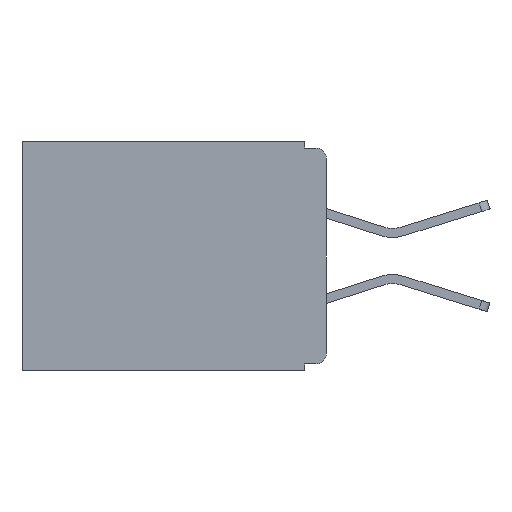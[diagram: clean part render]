
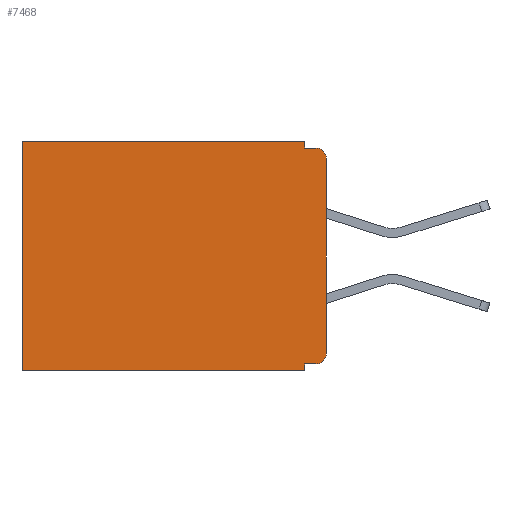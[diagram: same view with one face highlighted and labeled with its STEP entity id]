
A CAD part, left-side view. The second image highlights one B-rep face of the part: STEP entity #7468.
In plain terms, the highlighted planar face has unit normal (-1, 0, 0).
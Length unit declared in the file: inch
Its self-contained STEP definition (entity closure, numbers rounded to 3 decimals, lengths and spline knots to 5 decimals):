
#40 = CARTESIAN_POINT ( 'NONE',  ( 0.3, 0., -0.33 ) ) ;
#110 = CARTESIAN_POINT ( 'NONE',  ( 0.3, 0., -0.33 ) ) ;
#550 = VERTEX_POINT ( 'NONE', #2138 ) ;
#823 = ORIENTED_EDGE ( 'NONE', *, *, #13228, .T. ) ;
#982 = AXIS2_PLACEMENT_3D ( 'NONE', #19298, #19705, #19097 ) ;
#1581 = ORIENTED_EDGE ( 'NONE', *, *, #14726, .F. ) ;
#1845 = CARTESIAN_POINT ( 'NONE',  ( 0.3, 0., -0.32 ) ) ;
#2033 = AXIS2_PLACEMENT_3D ( 'NONE', #8565, #28020, #26029 ) ;
#2046 = DIRECTION ( 'NONE',  ( 0., 0., -1. ) ) ;
#2138 = CARTESIAN_POINT ( 'NONE',  ( 0.3, 0., -0.025 ) ) ;
#2230 = CARTESIAN_POINT ( 'NONE',  ( 0.3, 0.031, 0. ) ) ;
#2409 = EDGE_CURVE ( 'NONE', #550, #13899, #5448, .T. ) ;
#3191 = EDGE_CURVE ( 'NONE', #550, #28279, #14592, .T. ) ;
#3737 = EDGE_CURVE ( 'NONE', #4046, #18161, #4598, .T. ) ;
#4046 = VERTEX_POINT ( 'NONE', #23439 ) ;
#4598 = LINE ( 'NONE', #6097, #22523 ) ;
#5448 = LINE ( 'NONE', #110, #29412 ) ;
#5674 = CARTESIAN_POINT ( 'NONE',  ( 0.3, 0., -0.01 ) ) ;
#5685 = ORIENTED_EDGE ( 'NONE', *, *, #8941, .F. ) ;
#6097 = CARTESIAN_POINT ( 'NONE',  ( 0.3, 0.437, -0.33 ) ) ;
#6102 = ORIENTED_EDGE ( 'NONE', *, *, #2409, .F. ) ;
#6124 = DIRECTION ( 'NONE',  ( 0., 0., -1. ) ) ;
#6241 = EDGE_CURVE ( 'NONE', #25258, #23703, #10054, .T. ) ;
#6731 = ORIENTED_EDGE ( 'NONE', *, *, #9348, .F. ) ;
#7194 = CARTESIAN_POINT ( 'NONE',  ( 0.3, 0.015, -0.305 ) ) ;
#7468 = ADVANCED_FACE ( 'NONE', ( #25947 ), #19167, .F. ) ;
#7916 = CARTESIAN_POINT ( 'NONE',  ( 0.3, 0.031, -0.01 ) ) ;
#8565 = CARTESIAN_POINT ( 'NONE',  ( 0.3, 0.015, -0.025 ) ) ;
#8941 = EDGE_CURVE ( 'NONE', #23141, #21134, #21333, .T. ) ;
#9329 = CARTESIAN_POINT ( 'NONE',  ( 0.3, 0.031, -0.33 ) ) ;
#9348 = EDGE_CURVE ( 'NONE', #23703, #28279, #22755, .T. ) ;
#9586 = DIRECTION ( 'NONE',  ( 0., 0., -1. ) ) ;
#10054 = LINE ( 'NONE', #16228, #20951 ) ;
#10444 = DIRECTION ( 'NONE',  ( 0., -1., 0. ) ) ;
#10855 = VECTOR ( 'NONE', #18896, 39.37008 ) ;
#10928 = CARTESIAN_POINT ( 'NONE',  ( 0.3, 0., 0. ) ) ;
#11570 = LINE ( 'NONE', #40, #10855 ) ;
#11662 = DIRECTION ( 'NONE',  ( 0., 0., -1. ) ) ;
#11822 = VERTEX_POINT ( 'NONE', #27627 ) ;
#12008 = ORIENTED_EDGE ( 'NONE', *, *, #3191, .T. ) ;
#12976 = EDGE_CURVE ( 'NONE', #25258, #4046, #19289, .T. ) ;
#13106 = VECTOR ( 'NONE', #27158, 39.37008 ) ;
#13228 = EDGE_CURVE ( 'NONE', #23141, #13899, #29697, .T. ) ;
#13506 = ORIENTED_EDGE ( 'NONE', *, *, #3737, .T. ) ;
#13727 = VECTOR ( 'NONE', #11662, 39.37008 ) ;
#13899 = VERTEX_POINT ( 'NONE', #23688 ) ;
#14592 = CIRCLE ( 'NONE', #2033, 0.015 ) ;
#14726 = EDGE_CURVE ( 'NONE', #21134, #11822, #19909, .T. ) ;
#16228 = CARTESIAN_POINT ( 'NONE',  ( 0.3, 0.031, 0. ) ) ;
#16912 = CARTESIAN_POINT ( 'NONE',  ( 0.3, 0.015, -0.01 ) ) ;
#17722 = ORIENTED_EDGE ( 'NONE', *, *, #12976, .T. ) ;
#18161 = VERTEX_POINT ( 'NONE', #28253 ) ;
#18273 = DIRECTION ( 'NONE',  ( 0., 1., 0. ) ) ;
#18896 = DIRECTION ( 'NONE',  ( 0., 1., 0. ) ) ;
#19097 = DIRECTION ( 'NONE',  ( 0., 0., -1. ) ) ;
#19167 = PLANE ( 'NONE',  #982 ) ;
#19289 = LINE ( 'NONE', #10928, #13106 ) ;
#19298 = CARTESIAN_POINT ( 'NONE',  ( 0.3, 0., -0.33 ) ) ;
#19601 = EDGE_LOOP ( 'NONE', ( #6102, #12008, #6731, #24594, #17722, #13506, #25744, #1581, #5685, #823 ) ) ;
#19705 = DIRECTION ( 'NONE',  ( 1., 0., 0. ) ) ;
#19909 = LINE ( 'NONE', #9329, #13727 ) ;
#20597 = VECTOR ( 'NONE', #18273, 39.37008 ) ;
#20657 = CARTESIAN_POINT ( 'NONE',  ( 0.3, 0.015, -0.32 ) ) ;
#20951 = VECTOR ( 'NONE', #2046, 39.37008 ) ;
#21134 = VERTEX_POINT ( 'NONE', #27549 ) ;
#21333 = LINE ( 'NONE', #1845, #20597 ) ;
#21780 = AXIS2_PLACEMENT_3D ( 'NONE', #7194, #23515, #9586 ) ;
#22523 = VECTOR ( 'NONE', #6124, 39.37008 ) ;
#22755 = LINE ( 'NONE', #5674, #28177 ) ;
#23141 = VERTEX_POINT ( 'NONE', #20657 ) ;
#23361 = DIRECTION ( 'NONE',  ( 0., 0., -1. ) ) ;
#23439 = CARTESIAN_POINT ( 'NONE',  ( 0.3, 0.437, 0. ) ) ;
#23515 = DIRECTION ( 'NONE',  ( -1., 0., 0. ) ) ;
#23688 = CARTESIAN_POINT ( 'NONE',  ( 0.3, 0., -0.305 ) ) ;
#23703 = VERTEX_POINT ( 'NONE', #7916 ) ;
#24594 = ORIENTED_EDGE ( 'NONE', *, *, #6241, .F. ) ;
#25258 = VERTEX_POINT ( 'NONE', #2230 ) ;
#25744 = ORIENTED_EDGE ( 'NONE', *, *, #25972, .F. ) ;
#25947 = FACE_OUTER_BOUND ( 'NONE', #19601, .T. ) ;
#25972 = EDGE_CURVE ( 'NONE', #11822, #18161, #11570, .T. ) ;
#26029 = DIRECTION ( 'NONE',  ( 0., 0., -1. ) ) ;
#27158 = DIRECTION ( 'NONE',  ( 0., 1., 0. ) ) ;
#27549 = CARTESIAN_POINT ( 'NONE',  ( 0.3, 0.031, -0.32 ) ) ;
#27627 = CARTESIAN_POINT ( 'NONE',  ( 0.3, 0.031, -0.33 ) ) ;
#28020 = DIRECTION ( 'NONE',  ( -1., 0., 0. ) ) ;
#28177 = VECTOR ( 'NONE', #10444, 39.37008 ) ;
#28253 = CARTESIAN_POINT ( 'NONE',  ( 0.3, 0.437, -0.33 ) ) ;
#28279 = VERTEX_POINT ( 'NONE', #16912 ) ;
#29412 = VECTOR ( 'NONE', #23361, 39.37008 ) ;
#29697 = CIRCLE ( 'NONE', #21780, 0.015 ) ;
